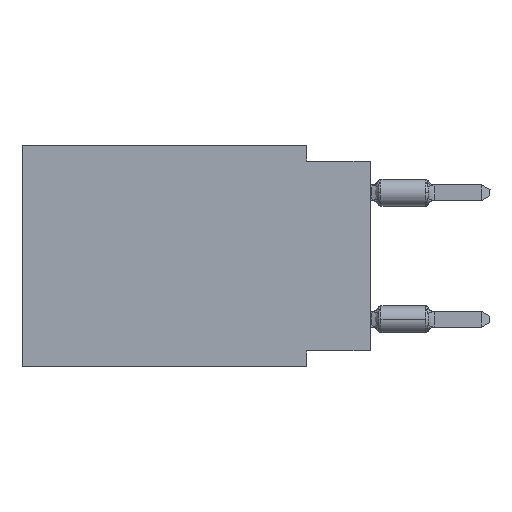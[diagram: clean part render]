
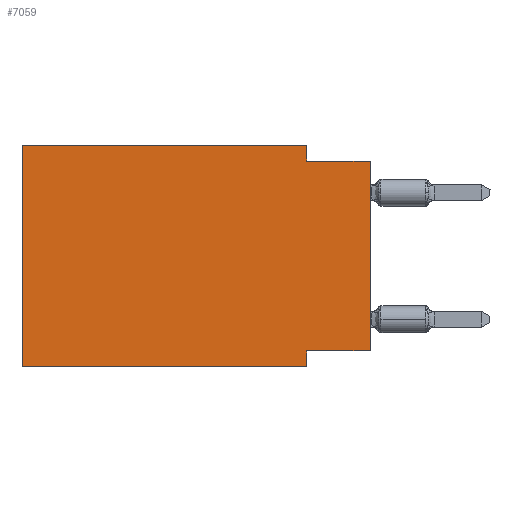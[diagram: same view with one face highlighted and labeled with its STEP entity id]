
A CAD part, left-side view. The second image highlights one B-rep face of the part: STEP entity #7059.
In plain terms, the highlighted planar face has unit normal (-1, 0, 0).
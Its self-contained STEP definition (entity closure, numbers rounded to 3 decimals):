
#476 = FACE_OUTER_BOUND ( 'NONE', #4411, .T. ) ;
#1361 = CARTESIAN_POINT ( 'NONE',  ( 0., 0., -0.635 ) ) ;
#1982 = LINE ( 'NONE', #25361, #14159 ) ;
#4132 = LINE ( 'NONE', #17577, #19967 ) ;
#4365 = CARTESIAN_POINT ( 'NONE',  ( 0., 13.97, -8.89 ) ) ;
#4411 = EDGE_LOOP ( 'NONE', ( #40776, #18386, #36652, #16483, #18207, #37449, #37516, #14467 ) ) ;
#4861 = LINE ( 'NONE', #24701, #43599 ) ;
#5093 = DIRECTION ( 'NONE',  ( 0., 1., 0. ) ) ;
#5708 = CARTESIAN_POINT ( 'NONE',  ( 0., 2.54, -8.89 ) ) ;
#5900 = EDGE_CURVE ( 'NONE', #38198, #12385, #29461, .T. ) ;
#7059 = ADVANCED_FACE ( 'NONE', ( #476 ), #13934, .F. ) ;
#7312 = DIRECTION ( 'NONE',  ( 0., 0., -1. ) ) ;
#9743 = CARTESIAN_POINT ( 'NONE',  ( 0., 2.54, -8.89 ) ) ;
#10633 = DIRECTION ( 'NONE',  ( 1., 0., 0. ) ) ;
#10634 = LINE ( 'NONE', #9743, #23814 ) ;
#11106 = LINE ( 'NONE', #17719, #12701 ) ;
#11798 = VERTEX_POINT ( 'NONE', #35311 ) ;
#12153 = DIRECTION ( 'NONE',  ( 0., -1., 0. ) ) ;
#12385 = VERTEX_POINT ( 'NONE', #5708 ) ;
#12701 = VECTOR ( 'NONE', #34477, 1000. ) ;
#12716 = CARTESIAN_POINT ( 'NONE',  ( 0., 13.97, -8.89 ) ) ;
#13934 = PLANE ( 'NONE',  #20625 ) ;
#14159 = VECTOR ( 'NONE', #5093, 1000. ) ;
#14467 = ORIENTED_EDGE ( 'NONE', *, *, #20123, .F. ) ;
#15737 = VECTOR ( 'NONE', #39003, 1000. ) ;
#16079 = VERTEX_POINT ( 'NONE', #16753 ) ;
#16081 = CARTESIAN_POINT ( 'NONE',  ( 0., 2.54, -8.255 ) ) ;
#16252 = EDGE_CURVE ( 'NONE', #38198, #11798, #18489, .T. ) ;
#16483 = ORIENTED_EDGE ( 'NONE', *, *, #37715, .F. ) ;
#16753 = CARTESIAN_POINT ( 'NONE',  ( 0., 2.54, 0. ) ) ;
#17577 = CARTESIAN_POINT ( 'NONE',  ( 0., 13.97, 0. ) ) ;
#17719 = CARTESIAN_POINT ( 'NONE',  ( 0., 0., 0. ) ) ;
#18207 = ORIENTED_EDGE ( 'NONE', *, *, #16252, .F. ) ;
#18259 = EDGE_CURVE ( 'NONE', #31101, #41380, #11106, .T. ) ;
#18386 = ORIENTED_EDGE ( 'NONE', *, *, #42348, .F. ) ;
#18489 = LINE ( 'NONE', #27971, #15737 ) ;
#18703 = EDGE_CURVE ( 'NONE', #16079, #34107, #4861, .T. ) ;
#19123 = DIRECTION ( 'NONE',  ( 0., -1., 0. ) ) ;
#19324 = CARTESIAN_POINT ( 'NONE',  ( 0., 2.54, -0.635 ) ) ;
#19967 = VECTOR ( 'NONE', #27714, 1000. ) ;
#20123 = EDGE_CURVE ( 'NONE', #31101, #20135, #1982, .T. ) ;
#20135 = VERTEX_POINT ( 'NONE', #16081 ) ;
#20625 = AXIS2_PLACEMENT_3D ( 'NONE', #27372, #10633, #27811 ) ;
#23186 = DIRECTION ( 'NONE',  ( 0., 0., -1. ) ) ;
#23814 = VECTOR ( 'NONE', #23186, 1000. ) ;
#24701 = CARTESIAN_POINT ( 'NONE',  ( 0., 2.54, 0. ) ) ;
#25189 = VECTOR ( 'NONE', #12153, 1000. ) ;
#25361 = CARTESIAN_POINT ( 'NONE',  ( 0., 0., -8.255 ) ) ;
#26169 = CARTESIAN_POINT ( 'NONE',  ( 0., 0., -8.255 ) ) ;
#27372 = CARTESIAN_POINT ( 'NONE',  ( 0., 13.97, 0. ) ) ;
#27714 = DIRECTION ( 'NONE',  ( 0., -1., 0. ) ) ;
#27811 = DIRECTION ( 'NONE',  ( 0., 0., -1. ) ) ;
#27971 = CARTESIAN_POINT ( 'NONE',  ( 0., 13.97, 0. ) ) ;
#29461 = LINE ( 'NONE', #12716, #38988 ) ;
#31101 = VERTEX_POINT ( 'NONE', #26169 ) ;
#31552 = LINE ( 'NONE', #1361, #25189 ) ;
#34107 = VERTEX_POINT ( 'NONE', #19324 ) ;
#34477 = DIRECTION ( 'NONE',  ( 0., 0., 1. ) ) ;
#34973 = EDGE_CURVE ( 'NONE', #20135, #12385, #10634, .T. ) ;
#35311 = CARTESIAN_POINT ( 'NONE',  ( 0., 13.97, 0. ) ) ;
#36652 = ORIENTED_EDGE ( 'NONE', *, *, #18703, .F. ) ;
#37449 = ORIENTED_EDGE ( 'NONE', *, *, #5900, .T. ) ;
#37516 = ORIENTED_EDGE ( 'NONE', *, *, #34973, .F. ) ;
#37715 = EDGE_CURVE ( 'NONE', #11798, #16079, #4132, .T. ) ;
#38198 = VERTEX_POINT ( 'NONE', #4365 ) ;
#38988 = VECTOR ( 'NONE', #19123, 1000. ) ;
#39003 = DIRECTION ( 'NONE',  ( 0., 0., 1. ) ) ;
#39823 = CARTESIAN_POINT ( 'NONE',  ( 0., 0., -0.635 ) ) ;
#40776 = ORIENTED_EDGE ( 'NONE', *, *, #18259, .T. ) ;
#41380 = VERTEX_POINT ( 'NONE', #39823 ) ;
#42348 = EDGE_CURVE ( 'NONE', #34107, #41380, #31552, .T. ) ;
#43599 = VECTOR ( 'NONE', #7312, 1000. ) ;
